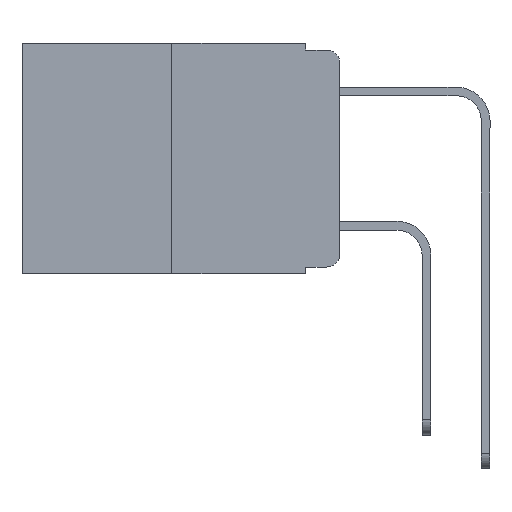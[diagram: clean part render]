
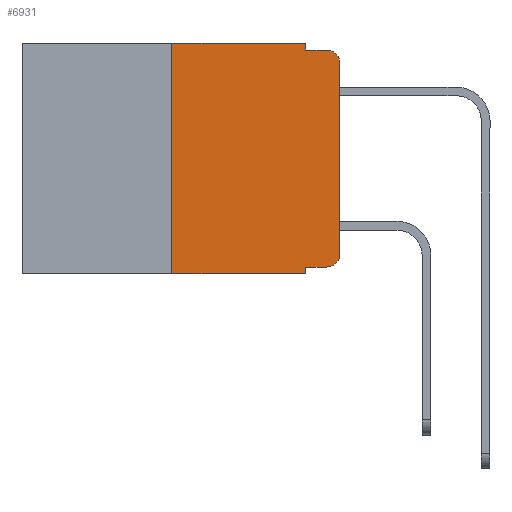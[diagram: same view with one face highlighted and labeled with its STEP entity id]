
A CAD part, left-side view. The second image highlights one B-rep face of the part: STEP entity #6931.
In plain terms, the highlighted planar face has unit normal (-1, 0, 0).
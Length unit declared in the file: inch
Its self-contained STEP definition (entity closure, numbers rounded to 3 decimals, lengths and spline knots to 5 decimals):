
#4 = ORIENTED_EDGE ( 'NONE', *, *, #8881, .T. ) ;
#121 = VERTEX_POINT ( 'NONE', #8233 ) ;
#148 = CARTESIAN_POINT ( 'NONE',  ( 0., 0.25, 0. ) ) ;
#352 = AXIS2_PLACEMENT_3D ( 'NONE', #6750, #6768, #10692 ) ;
#713 = CARTESIAN_POINT ( 'NONE',  ( 0., 0.051, -0.343 ) ) ;
#715 = DIRECTION ( 'NONE',  ( 0., 0., -1. ) ) ;
#979 = VERTEX_POINT ( 'NONE', #2111 ) ;
#983 = CIRCLE ( 'NONE', #4919, 0.02 ) ;
#1126 = CARTESIAN_POINT ( 'NONE',  ( 0., 0.051, 0. ) ) ;
#1144 = DIRECTION ( 'NONE',  ( 0., 0., -1. ) ) ;
#1388 = ORIENTED_EDGE ( 'NONE', *, *, #4119, .T. ) ;
#1477 = LINE ( 'NONE', #1126, #10976 ) ;
#1532 = VERTEX_POINT ( 'NONE', #10166 ) ;
#1573 = EDGE_CURVE ( 'NONE', #3517, #121, #10985, .T. ) ;
#1709 = VERTEX_POINT ( 'NONE', #6843 ) ;
#1777 = CARTESIAN_POINT ( 'NONE',  ( 0., 0.051, 0. ) ) ;
#1997 = VECTOR ( 'NONE', #8946, 39.37008 ) ;
#2027 = EDGE_CURVE ( 'NONE', #1709, #3517, #1477, .T. ) ;
#2111 = CARTESIAN_POINT ( 'NONE',  ( 0., 0., -0.313 ) ) ;
#2119 = ORIENTED_EDGE ( 'NONE', *, *, #6741, .T. ) ;
#2129 = CARTESIAN_POINT ( 'NONE',  ( 0., 0.051, -0.01 ) ) ;
#2735 = EDGE_CURVE ( 'NONE', #3709, #1709, #3996, .T. ) ;
#2800 = DIRECTION ( 'NONE',  ( -1., 0., 0. ) ) ;
#3379 = DIRECTION ( 'NONE',  ( 0., -1., 0. ) ) ;
#3517 = VERTEX_POINT ( 'NONE', #2129 ) ;
#3542 = EDGE_CURVE ( 'NONE', #3586, #7355, #4879, .T. ) ;
#3556 = VECTOR ( 'NONE', #8861, 39.37008 ) ;
#3586 = VERTEX_POINT ( 'NONE', #11066 ) ;
#3651 = DIRECTION ( 'NONE',  ( 0., 0., -1. ) ) ;
#3709 = VERTEX_POINT ( 'NONE', #148 ) ;
#3776 = ORIENTED_EDGE ( 'NONE', *, *, #7062, .F. ) ;
#3974 = CARTESIAN_POINT ( 'NONE',  ( 0., 0.051, -0.01 ) ) ;
#3996 = LINE ( 'NONE', #7208, #8500 ) ;
#4068 = VERTEX_POINT ( 'NONE', #6003 ) ;
#4119 = EDGE_CURVE ( 'NONE', #979, #4068, #8464, .T. ) ;
#4177 = ORIENTED_EDGE ( 'NONE', *, *, #2027, .F. ) ;
#4322 = DIRECTION ( 'NONE',  ( 0., -1., 0. ) ) ;
#4757 = DIRECTION ( 'NONE',  ( 0., 0., -1. ) ) ;
#4807 = ORIENTED_EDGE ( 'NONE', *, *, #8637, .T. ) ;
#4879 = LINE ( 'NONE', #1777, #9611 ) ;
#4919 = AXIS2_PLACEMENT_3D ( 'NONE', #7442, #11421, #3651 ) ;
#5072 = CARTESIAN_POINT ( 'NONE',  ( 0., 0., 0. ) ) ;
#5104 = VECTOR ( 'NONE', #3379, 39.37008 ) ;
#5111 = CARTESIAN_POINT ( 'NONE',  ( 0., 0.473, -0.343 ) ) ;
#5172 = EDGE_CURVE ( 'NONE', #4068, #121, #6668, .T. ) ;
#6003 = CARTESIAN_POINT ( 'NONE',  ( 0., 0., -0.03 ) ) ;
#6668 = CIRCLE ( 'NONE', #12278, 0.02 ) ;
#6741 = EDGE_CURVE ( 'NONE', #1532, #7355, #10079, .T. ) ;
#6744 = LINE ( 'NONE', #8640, #10969 ) ;
#6750 = CARTESIAN_POINT ( 'NONE',  ( 0., 0.473, 0. ) ) ;
#6768 = DIRECTION ( 'NONE',  ( 1., 0., 0. ) ) ;
#6843 = CARTESIAN_POINT ( 'NONE',  ( 0., 0.051, 0. ) ) ;
#6931 = ADVANCED_FACE ( 'NONE', ( #8388 ), #8349, .F. ) ;
#7046 = CARTESIAN_POINT ( 'NONE',  ( 0., 0.02, -0.03 ) ) ;
#7062 = EDGE_CURVE ( 'NONE', #1532, #3709, #11708, .T. ) ;
#7111 = ORIENTED_EDGE ( 'NONE', *, *, #3542, .F. ) ;
#7167 = CARTESIAN_POINT ( 'NONE',  ( 0., 0.02, -0.333 ) ) ;
#7208 = CARTESIAN_POINT ( 'NONE',  ( 0., 0.473, 0. ) ) ;
#7355 = VERTEX_POINT ( 'NONE', #713 ) ;
#7442 = CARTESIAN_POINT ( 'NONE',  ( 0., 0.02, -0.313 ) ) ;
#7617 = EDGE_LOOP ( 'NONE', ( #1388, #10241, #10111, #4177, #8591, #3776, #2119, #7111, #4, #4807 ) ) ;
#8035 = DIRECTION ( 'NONE',  ( 0., 0., 1. ) ) ;
#8233 = CARTESIAN_POINT ( 'NONE',  ( 0., 0.02, -0.01 ) ) ;
#8335 = DIRECTION ( 'NONE',  ( 0., -1., 0. ) ) ;
#8349 = PLANE ( 'NONE',  #352 ) ;
#8388 = FACE_OUTER_BOUND ( 'NONE', #7617, .T. ) ;
#8464 = LINE ( 'NONE', #5072, #10524 ) ;
#8500 = VECTOR ( 'NONE', #4322, 39.37008 ) ;
#8591 = ORIENTED_EDGE ( 'NONE', *, *, #2735, .F. ) ;
#8637 = EDGE_CURVE ( 'NONE', #11595, #979, #983, .T. ) ;
#8640 = CARTESIAN_POINT ( 'NONE',  ( 0., 0.051, -0.333 ) ) ;
#8861 = DIRECTION ( 'NONE',  ( 0., -1., 0. ) ) ;
#8881 = EDGE_CURVE ( 'NONE', #3586, #11595, #6744, .T. ) ;
#8946 = DIRECTION ( 'NONE',  ( 0., 0., 1. ) ) ;
#9611 = VECTOR ( 'NONE', #1144, 39.37008 ) ;
#10079 = LINE ( 'NONE', #5111, #5104 ) ;
#10111 = ORIENTED_EDGE ( 'NONE', *, *, #1573, .F. ) ;
#10166 = CARTESIAN_POINT ( 'NONE',  ( 0., 0.25, -0.343 ) ) ;
#10241 = ORIENTED_EDGE ( 'NONE', *, *, #5172, .T. ) ;
#10524 = VECTOR ( 'NONE', #8035, 39.37008 ) ;
#10692 = DIRECTION ( 'NONE',  ( 0., 0., -1. ) ) ;
#10969 = VECTOR ( 'NONE', #8335, 39.37008 ) ;
#10976 = VECTOR ( 'NONE', #715, 39.37008 ) ;
#10985 = LINE ( 'NONE', #3974, #3556 ) ;
#11066 = CARTESIAN_POINT ( 'NONE',  ( 0., 0.051, -0.333 ) ) ;
#11153 = CARTESIAN_POINT ( 'NONE',  ( 0., 0.25, 0. ) ) ;
#11421 = DIRECTION ( 'NONE',  ( -1., 0., 0. ) ) ;
#11595 = VERTEX_POINT ( 'NONE', #7167 ) ;
#11708 = LINE ( 'NONE', #11153, #1997 ) ;
#12278 = AXIS2_PLACEMENT_3D ( 'NONE', #7046, #2800, #4757 ) ;
